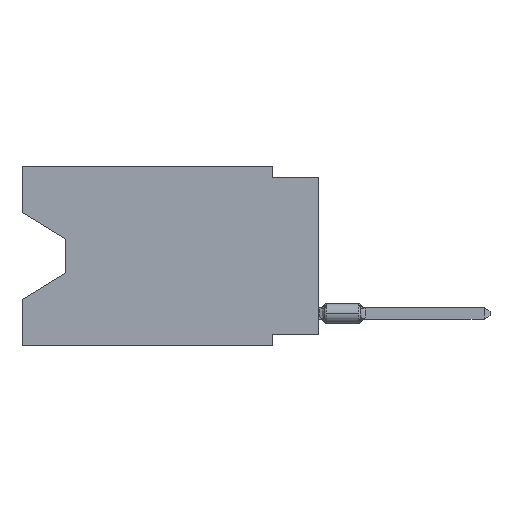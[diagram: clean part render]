
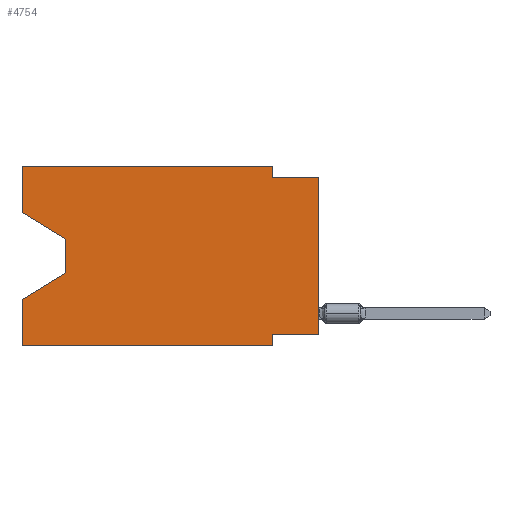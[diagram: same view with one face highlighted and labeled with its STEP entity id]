
A CAD part, left-side view. The second image highlights one B-rep face of the part: STEP entity #4754.
In plain terms, the highlighted planar face has unit normal (-1, 0, 0).
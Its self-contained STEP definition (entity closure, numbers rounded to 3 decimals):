
#70 = DIRECTION ( 'NONE',  ( 1., 0., 0. ) ) ;
#224 = CARTESIAN_POINT ( 'NONE',  ( 0., 0., -0.635 ) ) ;
#491 = CARTESIAN_POINT ( 'NONE',  ( 0., 2.54, 0. ) ) ;
#695 = VERTEX_POINT ( 'NONE', #11487 ) ;
#756 = ORIENTED_EDGE ( 'NONE', *, *, #5714, .F. ) ;
#792 = CARTESIAN_POINT ( 'NONE',  ( 0., 16.383, 0. ) ) ;
#1007 = VECTOR ( 'NONE', #5656, 1000. ) ;
#1021 = CARTESIAN_POINT ( 'NONE',  ( 0., 16.383, 0. ) ) ;
#1034 = DIRECTION ( 'NONE',  ( 0., 0., 1. ) ) ;
#1191 = VERTEX_POINT ( 'NONE', #12445 ) ;
#1290 = CARTESIAN_POINT ( 'NONE',  ( 0., 0., 0. ) ) ;
#1396 = EDGE_CURVE ( 'NONE', #7783, #4779, #9651, .T. ) ;
#1425 = LINE ( 'NONE', #6803, #1007 ) ;
#1490 = DIRECTION ( 'NONE',  ( 0., -1., 0. ) ) ;
#1665 = ORIENTED_EDGE ( 'NONE', *, *, #12472, .T. ) ;
#1791 = CARTESIAN_POINT ( 'NONE',  ( 0., 16.383, -7.36 ) ) ;
#1930 = EDGE_CURVE ( 'NONE', #13627, #14054, #7822, .T. ) ;
#1975 = DIRECTION ( 'NONE',  ( 0., 0., -1. ) ) ;
#2190 = EDGE_LOOP ( 'NONE', ( #11587, #9360, #4744, #756, #1665, #4023, #11109, #10553, #9258, #6612, #2699, #3023 ) ) ;
#2308 = VERTEX_POINT ( 'NONE', #792 ) ;
#2354 = CARTESIAN_POINT ( 'NONE',  ( 0., 0., -9.271 ) ) ;
#2450 = VERTEX_POINT ( 'NONE', #11468 ) ;
#2691 = VERTEX_POINT ( 'NONE', #1791 ) ;
#2699 = ORIENTED_EDGE ( 'NONE', *, *, #14189, .F. ) ;
#3023 = ORIENTED_EDGE ( 'NONE', *, *, #8390, .F. ) ;
#3504 = LINE ( 'NONE', #2354, #5379 ) ;
#3530 = EDGE_CURVE ( 'NONE', #1191, #10570, #3504, .T. ) ;
#3728 = EDGE_CURVE ( 'NONE', #2450, #13627, #5932, .T. ) ;
#4023 = ORIENTED_EDGE ( 'NONE', *, *, #13337, .F. ) ;
#4263 = CARTESIAN_POINT ( 'NONE',  ( 0., 16.383, 0. ) ) ;
#4519 = FACE_OUTER_BOUND ( 'NONE', #2190, .T. ) ;
#4635 = CARTESIAN_POINT ( 'NONE',  ( 0., 0., -0.635 ) ) ;
#4704 = CARTESIAN_POINT ( 'NONE',  ( 0., 13.97, -4.013 ) ) ;
#4734 = EDGE_CURVE ( 'NONE', #1191, #14054, #12133, .T. ) ;
#4735 = EDGE_CURVE ( 'NONE', #7447, #7783, #1425, .T. ) ;
#4744 = ORIENTED_EDGE ( 'NONE', *, *, #6552, .T. ) ;
#4754 = ADVANCED_FACE ( 'NONE', ( #4519 ), #10049, .F. ) ;
#4779 = VERTEX_POINT ( 'NONE', #13203 ) ;
#4947 = VECTOR ( 'NONE', #10152, 1000. ) ;
#4975 = LINE ( 'NONE', #13522, #9801 ) ;
#5379 = VECTOR ( 'NONE', #6724, 1000. ) ;
#5386 = DIRECTION ( 'NONE',  ( 0., 0., 1. ) ) ;
#5404 = VECTOR ( 'NONE', #9038, 1000. ) ;
#5460 = LINE ( 'NONE', #1021, #12846 ) ;
#5471 = LINE ( 'NONE', #4263, #6567 ) ;
#5656 = DIRECTION ( 'NONE',  ( 0., -0.855, -0.519 ) ) ;
#5714 = EDGE_CURVE ( 'NONE', #695, #2691, #5471, .T. ) ;
#5932 = LINE ( 'NONE', #491, #11605 ) ;
#6552 = EDGE_CURVE ( 'NONE', #4779, #2691, #6776, .T. ) ;
#6567 = VECTOR ( 'NONE', #1034, 1000. ) ;
#6612 = ORIENTED_EDGE ( 'NONE', *, *, #3728, .F. ) ;
#6724 = DIRECTION ( 'NONE',  ( 0., 1., 0. ) ) ;
#6776 = LINE ( 'NONE', #6984, #4947 ) ;
#6803 = CARTESIAN_POINT ( 'NONE',  ( 0., 16.383, -2.546 ) ) ;
#6984 = CARTESIAN_POINT ( 'NONE',  ( 0., 13.97, -5.893 ) ) ;
#7099 = CARTESIAN_POINT ( 'NONE',  ( 0., 2.54, -9.906 ) ) ;
#7148 = DIRECTION ( 'NONE',  ( 0., 0., -1. ) ) ;
#7447 = VERTEX_POINT ( 'NONE', #12606 ) ;
#7783 = VERTEX_POINT ( 'NONE', #4704 ) ;
#7822 = LINE ( 'NONE', #224, #10169 ) ;
#7833 = CARTESIAN_POINT ( 'NONE',  ( 0., 2.54, -0.635 ) ) ;
#7882 = DIRECTION ( 'NONE',  ( 0., 0., 1. ) ) ;
#7886 = CARTESIAN_POINT ( 'NONE',  ( 0., 16.383, -9.906 ) ) ;
#7965 = DIRECTION ( 'NONE',  ( 0., -1., 0. ) ) ;
#8131 = DIRECTION ( 'NONE',  ( 0., 0., -1. ) ) ;
#8318 = VECTOR ( 'NONE', #1975, 1000. ) ;
#8390 = EDGE_CURVE ( 'NONE', #7447, #2308, #5460, .T. ) ;
#9025 = AXIS2_PLACEMENT_3D ( 'NONE', #9033, #70, #13415 ) ;
#9033 = CARTESIAN_POINT ( 'NONE',  ( 0., 16.383, 0. ) ) ;
#9038 = DIRECTION ( 'NONE',  ( 0., -1., 0. ) ) ;
#9258 = ORIENTED_EDGE ( 'NONE', *, *, #1930, .F. ) ;
#9360 = ORIENTED_EDGE ( 'NONE', *, *, #1396, .T. ) ;
#9651 = LINE ( 'NONE', #14093, #8318 ) ;
#9801 = VECTOR ( 'NONE', #8131, 1000. ) ;
#10049 = PLANE ( 'NONE',  #9025 ) ;
#10152 = DIRECTION ( 'NONE',  ( 0., 0.855, -0.519 ) ) ;
#10169 = VECTOR ( 'NONE', #7965, 1000. ) ;
#10186 = LINE ( 'NONE', #7886, #5404 ) ;
#10526 = LINE ( 'NONE', #12671, #13178 ) ;
#10553 = ORIENTED_EDGE ( 'NONE', *, *, #4734, .T. ) ;
#10555 = CARTESIAN_POINT ( 'NONE',  ( 0., 2.54, -9.271 ) ) ;
#10570 = VERTEX_POINT ( 'NONE', #10555 ) ;
#11109 = ORIENTED_EDGE ( 'NONE', *, *, #3530, .F. ) ;
#11468 = CARTESIAN_POINT ( 'NONE',  ( 0., 2.54, 0. ) ) ;
#11487 = CARTESIAN_POINT ( 'NONE',  ( 0., 16.383, -9.906 ) ) ;
#11587 = ORIENTED_EDGE ( 'NONE', *, *, #4735, .T. ) ;
#11605 = VECTOR ( 'NONE', #7148, 1000. ) ;
#12133 = LINE ( 'NONE', #1290, #13384 ) ;
#12445 = CARTESIAN_POINT ( 'NONE',  ( 0., 0., -9.271 ) ) ;
#12472 = EDGE_CURVE ( 'NONE', #695, #13813, #10186, .T. ) ;
#12606 = CARTESIAN_POINT ( 'NONE',  ( 0., 16.383, -2.546 ) ) ;
#12671 = CARTESIAN_POINT ( 'NONE',  ( 0., 16.383, 0. ) ) ;
#12846 = VECTOR ( 'NONE', #5386, 1000. ) ;
#13178 = VECTOR ( 'NONE', #1490, 1000. ) ;
#13203 = CARTESIAN_POINT ( 'NONE',  ( 0., 13.97, -5.893 ) ) ;
#13337 = EDGE_CURVE ( 'NONE', #10570, #13813, #4975, .T. ) ;
#13384 = VECTOR ( 'NONE', #7882, 1000. ) ;
#13415 = DIRECTION ( 'NONE',  ( 0., 0., -1. ) ) ;
#13522 = CARTESIAN_POINT ( 'NONE',  ( 0., 2.54, -9.906 ) ) ;
#13627 = VERTEX_POINT ( 'NONE', #7833 ) ;
#13813 = VERTEX_POINT ( 'NONE', #7099 ) ;
#14054 = VERTEX_POINT ( 'NONE', #4635 ) ;
#14093 = CARTESIAN_POINT ( 'NONE',  ( 0., 13.97, -4.013 ) ) ;
#14189 = EDGE_CURVE ( 'NONE', #2308, #2450, #10526, .T. ) ;
